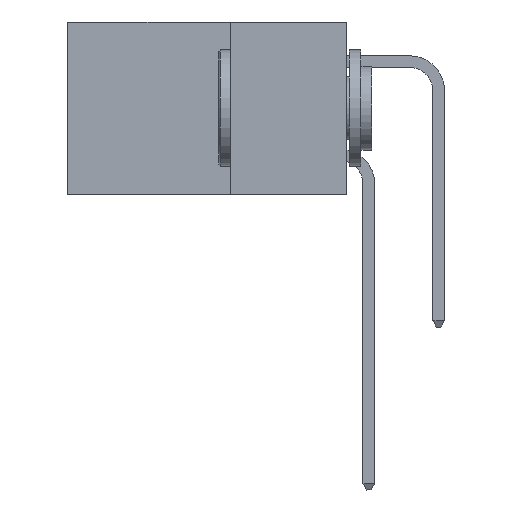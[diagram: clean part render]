
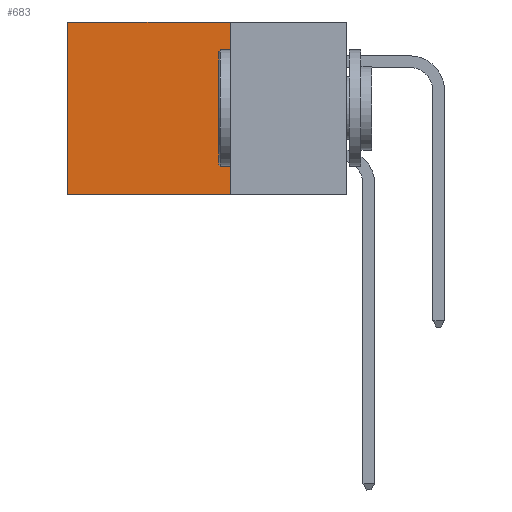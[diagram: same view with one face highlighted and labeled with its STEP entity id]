
A CAD part, left-side view. The second image highlights one B-rep face of the part: STEP entity #683.
In plain terms, the highlighted planar face has unit normal (-1, 0, 0).
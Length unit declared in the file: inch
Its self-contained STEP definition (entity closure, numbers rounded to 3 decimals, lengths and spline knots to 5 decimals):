
#683 = ADVANCED_FACE ( 'NONE', ( #1517 ), #1168, .F. ) ;
#859 = VECTOR ( 'NONE', #2131, 39.37008 ) ;
#1114 = DIRECTION ( 'NONE',  ( 0., 0., -1. ) ) ;
#1117 = DIRECTION ( 'NONE',  ( 1., 0., 0. ) ) ;
#1168 = PLANE ( 'NONE',  #19348 ) ;
#1271 = CARTESIAN_POINT ( 'NONE',  ( 0.2875, 0.25, 0. ) ) ;
#1291 = DIRECTION ( 'NONE',  ( 0., 0., -1. ) ) ;
#1517 = FACE_OUTER_BOUND ( 'NONE', #8199, .T. ) ;
#2039 = ORIENTED_EDGE ( 'NONE', *, *, #17878, .T. ) ;
#2131 = DIRECTION ( 'NONE',  ( 0., 1., 0. ) ) ;
#2692 = LINE ( 'NONE', #14588, #6790 ) ;
#3235 = EDGE_CURVE ( 'NONE', #11330, #16703, #5551, .T. ) ;
#3463 = CARTESIAN_POINT ( 'NONE',  ( 0.2875, 0.25, 0. ) ) ;
#3861 = ORIENTED_EDGE ( 'NONE', *, *, #3235, .F. ) ;
#3953 = VERTEX_POINT ( 'NONE', #7332 ) ;
#4989 = DIRECTION ( 'NONE',  ( 0., 1., 0. ) ) ;
#5191 = EDGE_CURVE ( 'NONE', #16703, #6036, #2692, .T. ) ;
#5551 = LINE ( 'NONE', #3463, #13548 ) ;
#6036 = VERTEX_POINT ( 'NONE', #11770 ) ;
#6790 = VECTOR ( 'NONE', #4989, 39.37008 ) ;
#7332 = CARTESIAN_POINT ( 'NONE',  ( 0.2875, 0.6, 0. ) ) ;
#8057 = CARTESIAN_POINT ( 'NONE',  ( 0.2875, 0.25, -0.37 ) ) ;
#8199 = EDGE_LOOP ( 'NONE', ( #2039, #12364, #3861, #16002 ) ) ;
#8942 = CARTESIAN_POINT ( 'NONE',  ( 0.2875, 0.25, 0. ) ) ;
#9250 = VECTOR ( 'NONE', #20330, 39.37008 ) ;
#9853 = LINE ( 'NONE', #10498, #859 ) ;
#10498 = CARTESIAN_POINT ( 'NONE',  ( 0.2875, 0.25, 0. ) ) ;
#11330 = VERTEX_POINT ( 'NONE', #8942 ) ;
#11770 = CARTESIAN_POINT ( 'NONE',  ( 0.2875, 0.6, -0.37 ) ) ;
#11995 = EDGE_CURVE ( 'NONE', #11330, #3953, #9853, .T. ) ;
#12364 = ORIENTED_EDGE ( 'NONE', *, *, #5191, .F. ) ;
#13548 = VECTOR ( 'NONE', #1291, 39.37008 ) ;
#14588 = CARTESIAN_POINT ( 'NONE',  ( 0.2875, 0.25, -0.37 ) ) ;
#16002 = ORIENTED_EDGE ( 'NONE', *, *, #11995, .T. ) ;
#16703 = VERTEX_POINT ( 'NONE', #8057 ) ;
#17609 = LINE ( 'NONE', #18781, #9250 ) ;
#17878 = EDGE_CURVE ( 'NONE', #3953, #6036, #17609, .T. ) ;
#18781 = CARTESIAN_POINT ( 'NONE',  ( 0.2875, 0.6, 0. ) ) ;
#19348 = AXIS2_PLACEMENT_3D ( 'NONE', #1271, #1117, #1114 ) ;
#20330 = DIRECTION ( 'NONE',  ( 0., 0., -1. ) ) ;
